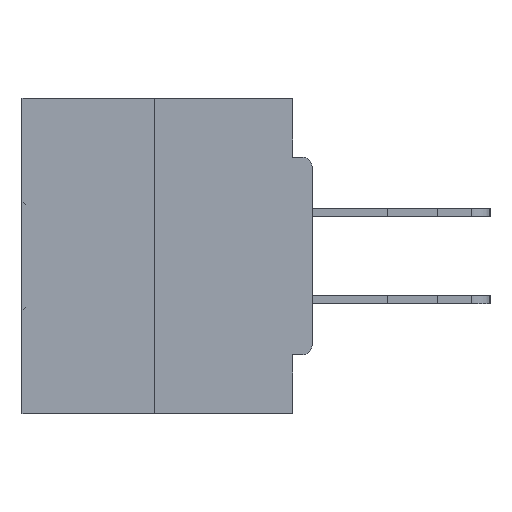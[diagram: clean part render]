
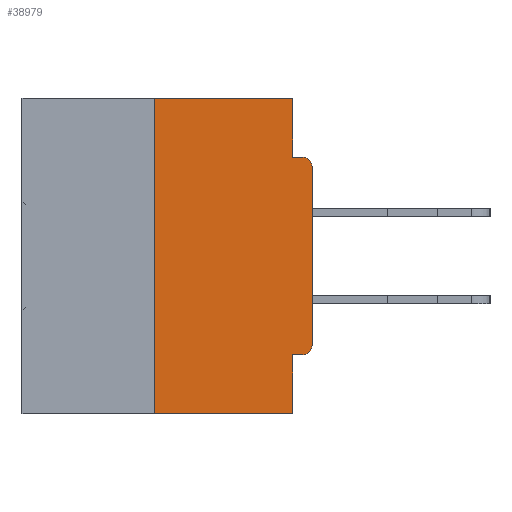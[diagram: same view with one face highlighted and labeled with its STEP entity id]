
A CAD part, left-side view. The second image highlights one B-rep face of the part: STEP entity #38979.
In plain terms, the highlighted planar face has unit normal (-1, 0, 0).
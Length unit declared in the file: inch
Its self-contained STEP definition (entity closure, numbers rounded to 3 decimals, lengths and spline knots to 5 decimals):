
#98 = DIRECTION ( 'NONE',  ( 0., -1., 0. ) ) ;
#189 = CARTESIAN_POINT ( 'NONE',  ( 0., 0.25, 0. ) ) ;
#224 = VERTEX_POINT ( 'NONE', #8720 ) ;
#1156 = ORIENTED_EDGE ( 'NONE', *, *, #14204, .F. ) ;
#1548 = DIRECTION ( 'NONE',  ( -1., 0., 0. ) ) ;
#1921 = VECTOR ( 'NONE', #34718, 39.37008 ) ;
#3526 = CARTESIAN_POINT ( 'NONE',  ( 0., 0.015, -0.4065 ) ) ;
#4010 = CARTESIAN_POINT ( 'NONE',  ( 0., 0., -0.0935 ) ) ;
#4932 = EDGE_CURVE ( 'NONE', #10134, #29440, #9149, .T. ) ;
#5463 = CARTESIAN_POINT ( 'NONE',  ( 0., 0.25, -0.5 ) ) ;
#6061 = DIRECTION ( 'NONE',  ( 0., -1., 0. ) ) ;
#6532 = CARTESIAN_POINT ( 'NONE',  ( 0., 0.031, -0.5 ) ) ;
#6615 = CIRCLE ( 'NONE', #30600, 0.015 ) ;
#7688 = LINE ( 'NONE', #9901, #39074 ) ;
#8720 = CARTESIAN_POINT ( 'NONE',  ( 0., 0.031, -0.4065 ) ) ;
#9137 = VERTEX_POINT ( 'NONE', #3526 ) ;
#9149 = LINE ( 'NONE', #4010, #33657 ) ;
#9458 = VERTEX_POINT ( 'NONE', #24253 ) ;
#9901 = CARTESIAN_POINT ( 'NONE',  ( 0., 0.46, -0.5 ) ) ;
#10134 = VERTEX_POINT ( 'NONE', #36608 ) ;
#10233 = ORIENTED_EDGE ( 'NONE', *, *, #32003, .F. ) ;
#10993 = DIRECTION ( 'NONE',  ( 0., 0., -1. ) ) ;
#12741 = CARTESIAN_POINT ( 'NONE',  ( 0., 0.46, 0. ) ) ;
#13239 = CARTESIAN_POINT ( 'NONE',  ( 0., 0.015, -0.0935 ) ) ;
#14204 = EDGE_CURVE ( 'NONE', #15730, #38207, #32819, .T. ) ;
#14486 = CARTESIAN_POINT ( 'NONE',  ( 0., 0.25, 0. ) ) ;
#14982 = DIRECTION ( 'NONE',  ( 0., 0., -1. ) ) ;
#15095 = DIRECTION ( 'NONE',  ( 0., 0., -1. ) ) ;
#15142 = ORIENTED_EDGE ( 'NONE', *, *, #36264, .F. ) ;
#15470 = EDGE_CURVE ( 'NONE', #9458, #10134, #30553, .T. ) ;
#15730 = VERTEX_POINT ( 'NONE', #5463 ) ;
#15897 = VECTOR ( 'NONE', #37803, 39.37008 ) ;
#16826 = ORIENTED_EDGE ( 'NONE', *, *, #27108, .T. ) ;
#18280 = DIRECTION ( 'NONE',  ( 1., 0., 0. ) ) ;
#18443 = EDGE_CURVE ( 'NONE', #41811, #29440, #6615, .T. ) ;
#19882 = DIRECTION ( 'NONE',  ( -1., 0., 0. ) ) ;
#21218 = AXIS2_PLACEMENT_3D ( 'NONE', #38660, #18280, #10993 ) ;
#21800 = ORIENTED_EDGE ( 'NONE', *, *, #30931, .T. ) ;
#21898 = EDGE_CURVE ( 'NONE', #41312, #41811, #42478, .T. ) ;
#23080 = VECTOR ( 'NONE', #6061, 39.37008 ) ;
#23700 = ORIENTED_EDGE ( 'NONE', *, *, #21898, .T. ) ;
#24253 = CARTESIAN_POINT ( 'NONE',  ( 0., 0.031, 0. ) ) ;
#25427 = VECTOR ( 'NONE', #15095, 39.37008 ) ;
#25515 = CARTESIAN_POINT ( 'NONE',  ( 0., 0.015, -0.3915 ) ) ;
#25784 = CARTESIAN_POINT ( 'NONE',  ( 0., 0., -0.1085 ) ) ;
#26574 = FACE_OUTER_BOUND ( 'NONE', #34212, .T. ) ;
#26721 = DIRECTION ( 'NONE',  ( 0., 0., -1. ) ) ;
#26816 = EDGE_CURVE ( 'NONE', #224, #42418, #34484, .T. ) ;
#26840 = VECTOR ( 'NONE', #34667, 39.37008 ) ;
#27108 = EDGE_CURVE ( 'NONE', #9137, #41312, #29086, .T. ) ;
#27176 = CARTESIAN_POINT ( 'NONE',  ( 0., 0., -0.4065 ) ) ;
#27503 = DIRECTION ( 'NONE',  ( 0., -1., 0. ) ) ;
#27537 = CARTESIAN_POINT ( 'NONE',  ( 0., 0.031, 0. ) ) ;
#29045 = ORIENTED_EDGE ( 'NONE', *, *, #18443, .T. ) ;
#29086 = CIRCLE ( 'NONE', #33985, 0.015 ) ;
#29440 = VERTEX_POINT ( 'NONE', #13239 ) ;
#30553 = LINE ( 'NONE', #27537, #26840 ) ;
#30600 = AXIS2_PLACEMENT_3D ( 'NONE', #40205, #19882, #26721 ) ;
#30931 = EDGE_CURVE ( 'NONE', #15730, #42418, #7688, .T. ) ;
#32003 = EDGE_CURVE ( 'NONE', #9137, #224, #42112, .T. ) ;
#32819 = LINE ( 'NONE', #14486, #1921 ) ;
#33657 = VECTOR ( 'NONE', #27503, 39.37008 ) ;
#33802 = ORIENTED_EDGE ( 'NONE', *, *, #4932, .F. ) ;
#33985 = AXIS2_PLACEMENT_3D ( 'NONE', #25515, #1548, #14982 ) ;
#34212 = EDGE_LOOP ( 'NONE', ( #15142, #1156, #21800, #37654, #10233, #16826, #23700, #29045, #33802, #41390 ) ) ;
#34386 = CARTESIAN_POINT ( 'NONE',  ( 0., 0., 0. ) ) ;
#34484 = LINE ( 'NONE', #35473, #25427 ) ;
#34667 = DIRECTION ( 'NONE',  ( 0., 0., -1. ) ) ;
#34718 = DIRECTION ( 'NONE',  ( 0., 0., 1. ) ) ;
#35473 = CARTESIAN_POINT ( 'NONE',  ( 0., 0.031, -0.5 ) ) ;
#36264 = EDGE_CURVE ( 'NONE', #38207, #9458, #41141, .T. ) ;
#36608 = CARTESIAN_POINT ( 'NONE',  ( 0., 0.031, -0.0935 ) ) ;
#37430 = DIRECTION ( 'NONE',  ( 0., 1., 0. ) ) ;
#37654 = ORIENTED_EDGE ( 'NONE', *, *, #26816, .F. ) ;
#37803 = DIRECTION ( 'NONE',  ( 0., 0., 1. ) ) ;
#37975 = CARTESIAN_POINT ( 'NONE',  ( 0., 0., -0.3915 ) ) ;
#38207 = VERTEX_POINT ( 'NONE', #189 ) ;
#38660 = CARTESIAN_POINT ( 'NONE',  ( 0., 0.46, 0. ) ) ;
#38979 = ADVANCED_FACE ( 'NONE', ( #26574 ), #41439, .F. ) ;
#39074 = VECTOR ( 'NONE', #98, 39.37008 ) ;
#40205 = CARTESIAN_POINT ( 'NONE',  ( 0., 0.015, -0.1085 ) ) ;
#41141 = LINE ( 'NONE', #12741, #23080 ) ;
#41312 = VERTEX_POINT ( 'NONE', #37975 ) ;
#41390 = ORIENTED_EDGE ( 'NONE', *, *, #15470, .F. ) ;
#41439 = PLANE ( 'NONE',  #21218 ) ;
#41557 = VECTOR ( 'NONE', #37430, 39.37008 ) ;
#41811 = VERTEX_POINT ( 'NONE', #25784 ) ;
#42112 = LINE ( 'NONE', #27176, #41557 ) ;
#42418 = VERTEX_POINT ( 'NONE', #6532 ) ;
#42478 = LINE ( 'NONE', #34386, #15897 ) ;
